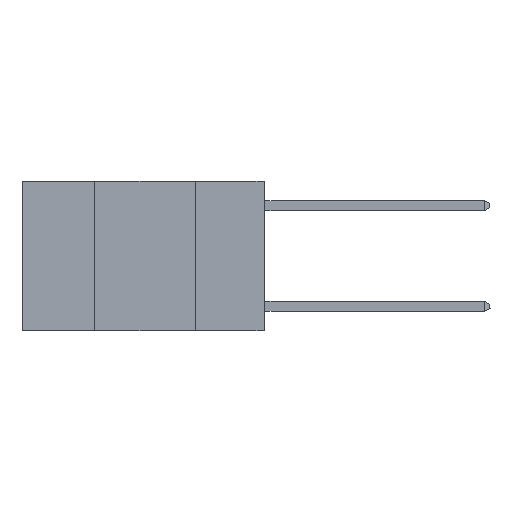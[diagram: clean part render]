
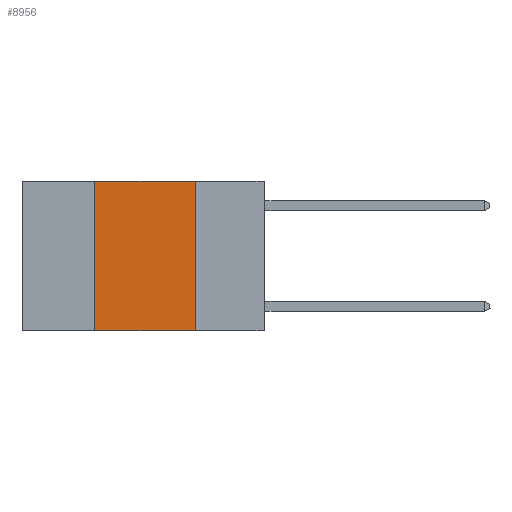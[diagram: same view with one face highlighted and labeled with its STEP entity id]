
A CAD part, left-side view. The second image highlights one B-rep face of the part: STEP entity #8956.
In plain terms, the highlighted planar face has unit normal (-1, 0, 0).
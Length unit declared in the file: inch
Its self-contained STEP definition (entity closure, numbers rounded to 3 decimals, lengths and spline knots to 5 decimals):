
#444 = AXIS2_PLACEMENT_3D ( 'NONE', #9283, #18453, #15570 ) ;
#577 = ORIENTED_EDGE ( 'NONE', *, *, #14361, .F. ) ;
#1112 = ORIENTED_EDGE ( 'NONE', *, *, #4666, .F. ) ;
#1496 = DIRECTION ( 'NONE',  ( 0., 0., 1. ) ) ;
#2383 = CARTESIAN_POINT ( 'NONE',  ( 0., 0.42, 0. ) ) ;
#2704 = ORIENTED_EDGE ( 'NONE', *, *, #12798, .F. ) ;
#2798 = VECTOR ( 'NONE', #1496, 39.37008 ) ;
#2976 = VERTEX_POINT ( 'NONE', #17128 ) ;
#3125 = CARTESIAN_POINT ( 'NONE',  ( 0., 0.17, 0. ) ) ;
#3782 = PLANE ( 'NONE',  #444 ) ;
#3802 = CARTESIAN_POINT ( 'NONE',  ( 0., 0.17, -0.37 ) ) ;
#4657 = DIRECTION ( 'NONE',  ( 0., 0., -1. ) ) ;
#4666 = EDGE_CURVE ( 'NONE', #17846, #17564, #16243, .T. ) ;
#6851 = ORIENTED_EDGE ( 'NONE', *, *, #13170, .T. ) ;
#8595 = CARTESIAN_POINT ( 'NONE',  ( 0., 0.42, 0. ) ) ;
#8792 = LINE ( 'NONE', #8595, #2798 ) ;
#8956 = ADVANCED_FACE ( 'NONE', ( #12607 ), #3782, .F. ) ;
#9283 = CARTESIAN_POINT ( 'NONE',  ( 0., 0.6, 0. ) ) ;
#10608 = CARTESIAN_POINT ( 'NONE',  ( 0., 0.17, 0. ) ) ;
#12607 = FACE_OUTER_BOUND ( 'NONE', #17541, .T. ) ;
#12798 = EDGE_CURVE ( 'NONE', #17530, #17846, #13623, .T. ) ;
#13170 = EDGE_CURVE ( 'NONE', #2976, #17564, #16181, .T. ) ;
#13482 = VECTOR ( 'NONE', #16777, 39.37008 ) ;
#13623 = LINE ( 'NONE', #16680, #13482 ) ;
#14080 = VECTOR ( 'NONE', #14745, 39.37008 ) ;
#14361 = EDGE_CURVE ( 'NONE', #2976, #17530, #8792, .T. ) ;
#14745 = DIRECTION ( 'NONE',  ( 0., -1., 0. ) ) ;
#15570 = DIRECTION ( 'NONE',  ( 0., 0., -1. ) ) ;
#16181 = LINE ( 'NONE', #17344, #14080 ) ;
#16243 = LINE ( 'NONE', #3125, #16853 ) ;
#16680 = CARTESIAN_POINT ( 'NONE',  ( 0., 0.6, 0. ) ) ;
#16777 = DIRECTION ( 'NONE',  ( 0., -1., 0. ) ) ;
#16853 = VECTOR ( 'NONE', #4657, 39.37008 ) ;
#17128 = CARTESIAN_POINT ( 'NONE',  ( 0., 0.42, -0.37 ) ) ;
#17344 = CARTESIAN_POINT ( 'NONE',  ( 0., 0.6, -0.37 ) ) ;
#17530 = VERTEX_POINT ( 'NONE', #2383 ) ;
#17541 = EDGE_LOOP ( 'NONE', ( #1112, #2704, #577, #6851 ) ) ;
#17564 = VERTEX_POINT ( 'NONE', #3802 ) ;
#17846 = VERTEX_POINT ( 'NONE', #10608 ) ;
#18453 = DIRECTION ( 'NONE',  ( 1., 0., 0. ) ) ;
